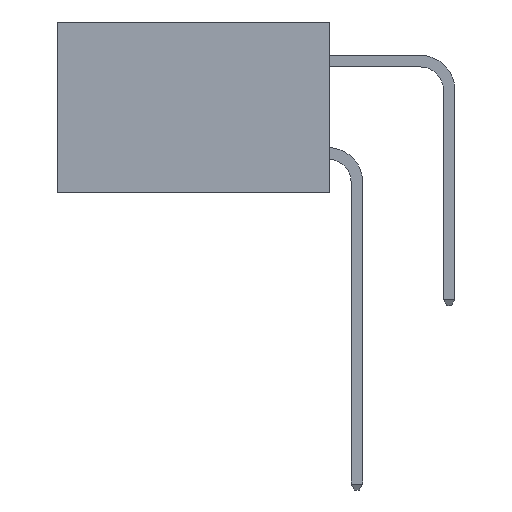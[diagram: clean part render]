
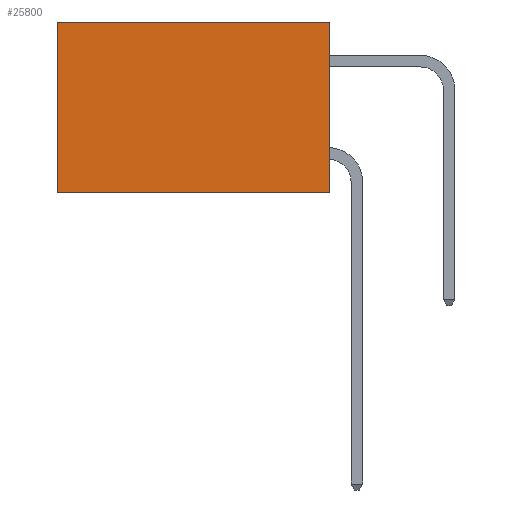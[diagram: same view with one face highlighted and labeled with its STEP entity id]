
A CAD part, left-side view. The second image highlights one B-rep face of the part: STEP entity #25800.
In plain terms, the highlighted planar face has unit normal (-1, 0, 0).
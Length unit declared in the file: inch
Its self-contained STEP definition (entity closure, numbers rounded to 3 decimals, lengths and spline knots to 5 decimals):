
#429 = VECTOR ( 'NONE', #16064, 39.37008 ) ;
#472 = CARTESIAN_POINT ( 'NONE',  ( 0.277, 0.59, -0.37 ) ) ;
#1108 = PLANE ( 'NONE',  #22929 ) ;
#1708 = VERTEX_POINT ( 'NONE', #29347 ) ;
#1986 = CARTESIAN_POINT ( 'NONE',  ( 0.277, 0., 0. ) ) ;
#3319 = FACE_OUTER_BOUND ( 'NONE', #15529, .T. ) ;
#5001 = LINE ( 'NONE', #6636, #11140 ) ;
#6264 = VERTEX_POINT ( 'NONE', #22427 ) ;
#6636 = CARTESIAN_POINT ( 'NONE',  ( 0.277, 0., 0. ) ) ;
#8974 = DIRECTION ( 'NONE',  ( 1., 0., 0. ) ) ;
#9665 = CARTESIAN_POINT ( 'NONE',  ( 0.277, 0., -0.37 ) ) ;
#11140 = VECTOR ( 'NONE', #29570, 39.37008 ) ;
#12340 = DIRECTION ( 'NONE',  ( 0., 1., 0. ) ) ;
#12757 = VECTOR ( 'NONE', #24867, 39.37008 ) ;
#12797 = EDGE_CURVE ( 'NONE', #26593, #29473, #5001, .T. ) ;
#12969 = ORIENTED_EDGE ( 'NONE', *, *, #18365, .T. ) ;
#15090 = VECTOR ( 'NONE', #12340, 39.37008 ) ;
#15529 = EDGE_LOOP ( 'NONE', ( #12969, #20303, #22980, #22257 ) ) ;
#15901 = LINE ( 'NONE', #17455, #15090 ) ;
#16064 = DIRECTION ( 'NONE',  ( 0., 0., -1. ) ) ;
#17455 = CARTESIAN_POINT ( 'NONE',  ( 0.277, 0., -0.37 ) ) ;
#18365 = EDGE_CURVE ( 'NONE', #29473, #1708, #21040, .T. ) ;
#19521 = LINE ( 'NONE', #9665, #12757 ) ;
#20303 = ORIENTED_EDGE ( 'NONE', *, *, #25302, .F. ) ;
#21040 = LINE ( 'NONE', #472, #429 ) ;
#22257 = ORIENTED_EDGE ( 'NONE', *, *, #12797, .T. ) ;
#22427 = CARTESIAN_POINT ( 'NONE',  ( 0.277, 0., -0.37 ) ) ;
#22929 = AXIS2_PLACEMENT_3D ( 'NONE', #24222, #8974, #26754 ) ;
#22980 = ORIENTED_EDGE ( 'NONE', *, *, #29931, .F. ) ;
#24222 = CARTESIAN_POINT ( 'NONE',  ( 0.277, 0., -0.37 ) ) ;
#24867 = DIRECTION ( 'NONE',  ( 0., 0., -1. ) ) ;
#25302 = EDGE_CURVE ( 'NONE', #6264, #1708, #15901, .T. ) ;
#25335 = CARTESIAN_POINT ( 'NONE',  ( 0.277, 0.59, 0. ) ) ;
#25800 = ADVANCED_FACE ( 'NONE', ( #3319 ), #1108, .F. ) ;
#26593 = VERTEX_POINT ( 'NONE', #1986 ) ;
#26754 = DIRECTION ( 'NONE',  ( 0., 0., -1. ) ) ;
#29347 = CARTESIAN_POINT ( 'NONE',  ( 0.277, 0.59, -0.37 ) ) ;
#29473 = VERTEX_POINT ( 'NONE', #25335 ) ;
#29570 = DIRECTION ( 'NONE',  ( 0., 1., 0. ) ) ;
#29931 = EDGE_CURVE ( 'NONE', #26593, #6264, #19521, .T. ) ;
